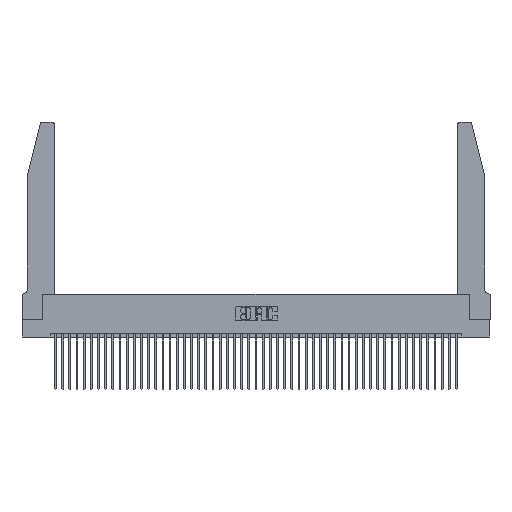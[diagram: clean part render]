
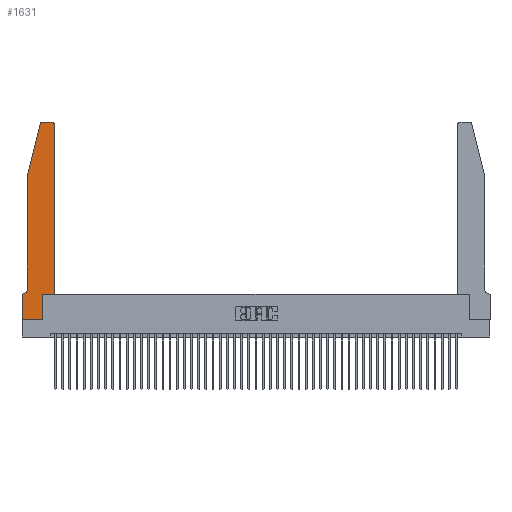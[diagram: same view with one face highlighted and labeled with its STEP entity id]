
A CAD part, top view. The second image highlights one B-rep face of the part: STEP entity #1631.
In plain terms, the highlighted planar face has unit normal (0, 0, 1).
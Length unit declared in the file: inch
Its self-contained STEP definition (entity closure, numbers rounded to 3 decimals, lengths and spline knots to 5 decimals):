
#408 = ORIENTED_EDGE ( 'NONE', *, *, #26321, .T. ) ;
#640 = LINE ( 'NONE', #21559, #15628 ) ;
#1283 = EDGE_CURVE ( 'NONE', #21591, #2341, #5801, .T. ) ;
#1631 = ADVANCED_FACE ( 'NONE', ( #23555 ), #17329, .T. ) ;
#1637 = CARTESIAN_POINT ( 'NONE',  ( 0.0755, 2., 0.37 ) ) ;
#2066 = CARTESIAN_POINT ( 'NONE',  ( 0., 0.35, 0.37 ) ) ;
#2341 = VERTEX_POINT ( 'NONE', #3145 ) ;
#2838 = DIRECTION ( 'NONE',  ( -1., 0., 0. ) ) ;
#3145 = CARTESIAN_POINT ( 'NONE',  ( 0.4505, 2.72, 0.37 ) ) ;
#3533 = LINE ( 'NONE', #27832, #28173 ) ;
#3616 = CARTESIAN_POINT ( 'NONE',  ( 0.4205, 2.72, 0.37 ) ) ;
#3741 = VECTOR ( 'NONE', #35748, 39.37008 ) ;
#4280 = ORIENTED_EDGE ( 'NONE', *, *, #29985, .T. ) ;
#4517 = ORIENTED_EDGE ( 'NONE', *, *, #37116, .T. ) ;
#5467 = VERTEX_POINT ( 'NONE', #17212 ) ;
#5635 = CARTESIAN_POINT ( 'NONE',  ( 0.284, 2.72, 0.37 ) ) ;
#5801 = LINE ( 'NONE', #11036, #21852 ) ;
#6929 = CARTESIAN_POINT ( 'NONE',  ( 0.284, 2.75, 0.37 ) ) ;
#7341 = CIRCLE ( 'NONE', #24454, 0.07 ) ;
#7439 = VERTEX_POINT ( 'NONE', #43239 ) ;
#8303 = CARTESIAN_POINT ( 'NONE',  ( 0.0755, 0.42, 0.37 ) ) ;
#9257 = CIRCLE ( 'NONE', #16979, 0.03 ) ;
#10723 = VERTEX_POINT ( 'NONE', #1637 ) ;
#11036 = CARTESIAN_POINT ( 'NONE',  ( 0.4505, 0.35, 0.37 ) ) ;
#11753 = EDGE_CURVE ( 'NONE', #10723, #12147, #38708, .T. ) ;
#12147 = VERTEX_POINT ( 'NONE', #8303 ) ;
#12554 = DIRECTION ( 'NONE',  ( 1., 0., 0. ) ) ;
#12960 = CARTESIAN_POINT ( 'NONE',  ( 0.0755, 2., 0.37 ) ) ;
#13398 = LINE ( 'NONE', #27151, #35767 ) ;
#13447 = EDGE_LOOP ( 'NONE', ( #16269, #15089, #27723, #43990, #408, #25389, #35883, #19743, #20896, #4280, #38044, #4517 ) ) ;
#13604 = CARTESIAN_POINT ( 'NONE',  ( 0.25487, 2.72718, 0.37 ) ) ;
#14210 = DIRECTION ( 'NONE',  ( 0., 1., 0. ) ) ;
#14536 = VECTOR ( 'NONE', #29485, 39.37008 ) ;
#14812 = DIRECTION ( 'NONE',  ( 1., 0., 0. ) ) ;
#14968 = EDGE_CURVE ( 'NONE', #45846, #21045, #28702, .T. ) ;
#15089 = ORIENTED_EDGE ( 'NONE', *, *, #35552, .T. ) ;
#15628 = VECTOR ( 'NONE', #2838, 39.37008 ) ;
#16269 = ORIENTED_EDGE ( 'NONE', *, *, #23202, .T. ) ;
#16288 = EDGE_CURVE ( 'NONE', #7439, #19727, #25832, .T. ) ;
#16292 = DIRECTION ( 'NONE',  ( 1., 0., 0. ) ) ;
#16342 = CARTESIAN_POINT ( 'NONE',  ( 0.4505, 0.35, 0.37 ) ) ;
#16625 = VECTOR ( 'NONE', #40724, 39.37008 ) ;
#16979 = AXIS2_PLACEMENT_3D ( 'NONE', #5635, #38003, #41841 ) ;
#17212 = CARTESIAN_POINT ( 'NONE',  ( 0.0055, 0.35, 0.37 ) ) ;
#17329 = PLANE ( 'NONE',  #38937 ) ;
#17615 = AXIS2_PLACEMENT_3D ( 'NONE', #3616, #22023, #14812 ) ;
#19727 = VERTEX_POINT ( 'NONE', #34718 ) ;
#19743 = ORIENTED_EDGE ( 'NONE', *, *, #43623, .T. ) ;
#20896 = ORIENTED_EDGE ( 'NONE', *, *, #16288, .T. ) ;
#21045 = VERTEX_POINT ( 'NONE', #36042 ) ;
#21559 = CARTESIAN_POINT ( 'NONE',  ( 0.0755, 0.35, 0.37 ) ) ;
#21591 = VERTEX_POINT ( 'NONE', #16342 ) ;
#21668 = CARTESIAN_POINT ( 'NONE',  ( 0.0755, 2., 0.37 ) ) ;
#21852 = VECTOR ( 'NONE', #14210, 39.37008 ) ;
#22023 = DIRECTION ( 'NONE',  ( 0., 0., 1. ) ) ;
#23202 = EDGE_CURVE ( 'NONE', #28518, #33427, #44854, .T. ) ;
#23442 = DIRECTION ( 'NONE',  ( 0., 0., -1. ) ) ;
#23555 = FACE_OUTER_BOUND ( 'NONE', #13447, .T. ) ;
#24454 = AXIS2_PLACEMENT_3D ( 'NONE', #45888, #23442, #42345 ) ;
#25389 = ORIENTED_EDGE ( 'NONE', *, *, #44559, .T. ) ;
#25832 = LINE ( 'NONE', #38208, #45923 ) ;
#26321 = EDGE_CURVE ( 'NONE', #12147, #5467, #7341, .T. ) ;
#26743 = CARTESIAN_POINT ( 'NONE',  ( 0., 0., 0.37 ) ) ;
#27151 = CARTESIAN_POINT ( 'NONE',  ( 0., 0., 0.37 ) ) ;
#27723 = ORIENTED_EDGE ( 'NONE', *, *, #40187, .T. ) ;
#27832 = CARTESIAN_POINT ( 'NONE',  ( 0.4505, 0.35, 0.37 ) ) ;
#28173 = VECTOR ( 'NONE', #16292, 39.37008 ) ;
#28518 = VERTEX_POINT ( 'NONE', #29037 ) ;
#28702 = LINE ( 'NONE', #26743, #16625 ) ;
#29037 = CARTESIAN_POINT ( 'NONE',  ( 0.4205, 2.75, 0.37 ) ) ;
#29485 = DIRECTION ( 'NONE',  ( -0.239, -0.971, 0. ) ) ;
#29985 = EDGE_CURVE ( 'NONE', #19727, #21591, #3533, .T. ) ;
#31101 = VECTOR ( 'NONE', #32687, 39.37008 ) ;
#31777 = DIRECTION ( 'NONE',  ( 1., 0., 0. ) ) ;
#32687 = DIRECTION ( 'NONE',  ( -1., 0., 0. ) ) ;
#32846 = CARTESIAN_POINT ( 'NONE',  ( 0.2605, 2.75, 0.37 ) ) ;
#33427 = VERTEX_POINT ( 'NONE', #6929 ) ;
#34718 = CARTESIAN_POINT ( 'NONE',  ( 0.2865, 0.35, 0.37 ) ) ;
#35552 = EDGE_CURVE ( 'NONE', #33427, #40611, #9257, .T. ) ;
#35748 = DIRECTION ( 'NONE',  ( 0., -1., 0. ) ) ;
#35767 = VECTOR ( 'NONE', #12554, 39.37008 ) ;
#35883 = ORIENTED_EDGE ( 'NONE', *, *, #14968, .T. ) ;
#36042 = CARTESIAN_POINT ( 'NONE',  ( 0., 0., 0.37 ) ) ;
#37116 = EDGE_CURVE ( 'NONE', #2341, #28518, #37181, .T. ) ;
#37181 = CIRCLE ( 'NONE', #17615, 0.03 ) ;
#37579 = DIRECTION ( 'NONE',  ( 0., 1., 0. ) ) ;
#38003 = DIRECTION ( 'NONE',  ( 0., 0., 1. ) ) ;
#38044 = ORIENTED_EDGE ( 'NONE', *, *, #1283, .T. ) ;
#38208 = CARTESIAN_POINT ( 'NONE',  ( 0.2865, 0.35, 0.37 ) ) ;
#38708 = LINE ( 'NONE', #12960, #3741 ) ;
#38937 = AXIS2_PLACEMENT_3D ( 'NONE', #46045, #42969, #31777 ) ;
#40187 = EDGE_CURVE ( 'NONE', #40611, #10723, #45468, .T. ) ;
#40611 = VERTEX_POINT ( 'NONE', #13604 ) ;
#40724 = DIRECTION ( 'NONE',  ( 0., -1., 0. ) ) ;
#41841 = DIRECTION ( 'NONE',  ( 1., 0., 0. ) ) ;
#42345 = DIRECTION ( 'NONE',  ( -1., 0., 0. ) ) ;
#42969 = DIRECTION ( 'NONE',  ( 0., 0., 1. ) ) ;
#43239 = CARTESIAN_POINT ( 'NONE',  ( 0.2865, 0., 0.37 ) ) ;
#43623 = EDGE_CURVE ( 'NONE', #21045, #7439, #13398, .T. ) ;
#43990 = ORIENTED_EDGE ( 'NONE', *, *, #11753, .T. ) ;
#44559 = EDGE_CURVE ( 'NONE', #5467, #45846, #640, .T. ) ;
#44854 = LINE ( 'NONE', #32846, #31101 ) ;
#45468 = LINE ( 'NONE', #21668, #14536 ) ;
#45846 = VERTEX_POINT ( 'NONE', #2066 ) ;
#45888 = CARTESIAN_POINT ( 'NONE',  ( 0.0055, 0.42, 0.37 ) ) ;
#45923 = VECTOR ( 'NONE', #37579, 39.37008 ) ;
#46045 = CARTESIAN_POINT ( 'NONE',  ( 0., 0.35, 0.37 ) ) ;
